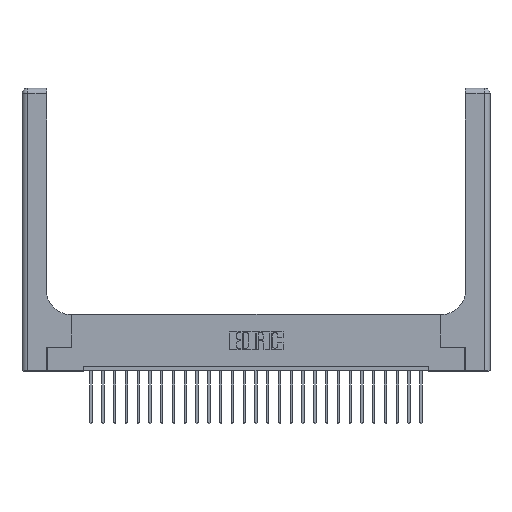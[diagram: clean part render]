
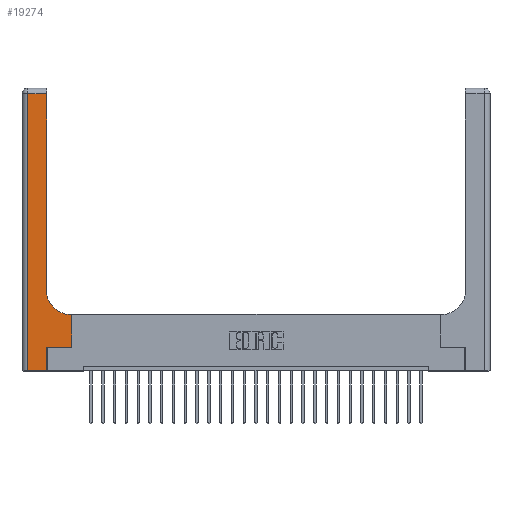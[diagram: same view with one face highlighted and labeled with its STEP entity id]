
A CAD part, top view. The second image highlights one B-rep face of the part: STEP entity #19274.
In plain terms, the highlighted planar face has unit normal (0, 0, 1).
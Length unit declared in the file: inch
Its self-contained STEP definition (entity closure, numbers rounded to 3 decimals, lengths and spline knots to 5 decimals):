
#1393 = CARTESIAN_POINT ( 'NONE',  ( 0., 0., 0.37 ) ) ;
#2733 = VERTEX_POINT ( 'NONE', #12878 ) ;
#2893 = EDGE_CURVE ( 'NONE', #7066, #9478, #19271, .T. ) ;
#3569 = CARTESIAN_POINT ( 'NONE',  ( 0., 2.94, 0.37 ) ) ;
#3649 = CARTESIAN_POINT ( 'NONE',  ( 0.51, 0.6, 0.37 ) ) ;
#3749 = EDGE_CURVE ( 'NONE', #22041, #7944, #23563, .T. ) ;
#4116 = CARTESIAN_POINT ( 'NONE',  ( 0., 3., 0.37 ) ) ;
#4631 = EDGE_CURVE ( 'NONE', #9478, #13828, #14816, .T. ) ;
#4731 = CARTESIAN_POINT ( 'NONE',  ( 0.528, 0.25, 0.37 ) ) ;
#5255 = LINE ( 'NONE', #1393, #12780 ) ;
#5630 = CIRCLE ( 'NONE', #20385, 0.25 ) ;
#5872 = DIRECTION ( 'NONE',  ( -1., 0., 0. ) ) ;
#5969 = DIRECTION ( 'NONE',  ( 0., 1., 0. ) ) ;
#6547 = EDGE_CURVE ( 'NONE', #13828, #21429, #15803, .T. ) ;
#6646 = DIRECTION ( 'NONE',  ( 1., 0., 0. ) ) ;
#6656 = CARTESIAN_POINT ( 'NONE',  ( 0.265, 0.25, 0.37 ) ) ;
#6867 = EDGE_CURVE ( 'NONE', #2733, #7066, #20140, .T. ) ;
#7066 = VERTEX_POINT ( 'NONE', #6656 ) ;
#7307 = DIRECTION ( 'NONE',  ( 1., 0., 0. ) ) ;
#7593 = CARTESIAN_POINT ( 'NONE',  ( 0.265, 0.25, 0.37 ) ) ;
#7886 = AXIS2_PLACEMENT_3D ( 'NONE', #4116, #15931, #19772 ) ;
#7944 = VERTEX_POINT ( 'NONE', #18975 ) ;
#8501 = ORIENTED_EDGE ( 'NONE', *, *, #2893, .T. ) ;
#8572 = CARTESIAN_POINT ( 'NONE',  ( 0.51, 0.85, 0.37 ) ) ;
#8751 = VECTOR ( 'NONE', #16295, 39.37008 ) ;
#9478 = VERTEX_POINT ( 'NONE', #4731 ) ;
#10160 = DIRECTION ( 'NONE',  ( -1., 0., 0. ) ) ;
#10286 = FACE_OUTER_BOUND ( 'NONE', #10480, .T. ) ;
#10480 = EDGE_LOOP ( 'NONE', ( #19720, #17516, #15039, #15432, #15821, #8501, #23586, #16377, #21951 ) ) ;
#10783 = VERTEX_POINT ( 'NONE', #24390 ) ;
#10808 = VECTOR ( 'NONE', #5969, 39.37008 ) ;
#11617 = VECTOR ( 'NONE', #14775, 39.37008 ) ;
#11956 = CARTESIAN_POINT ( 'NONE',  ( 0.26, 0.6, 0.37 ) ) ;
#12054 = CARTESIAN_POINT ( 'NONE',  ( 0.265, 0., 0.37 ) ) ;
#12780 = VECTOR ( 'NONE', #7307, 39.37008 ) ;
#12878 = CARTESIAN_POINT ( 'NONE',  ( 0.265, 0., 0.37 ) ) ;
#12920 = CARTESIAN_POINT ( 'NONE',  ( 0.528, 0.6, 0.37 ) ) ;
#13828 = VERTEX_POINT ( 'NONE', #12920 ) ;
#14417 = VECTOR ( 'NONE', #14699, 39.37008 ) ;
#14699 = DIRECTION ( 'NONE',  ( 0., 1., 0. ) ) ;
#14775 = DIRECTION ( 'NONE',  ( 0., -1., 0. ) ) ;
#14816 = LINE ( 'NONE', #16756, #14417 ) ;
#14889 = LINE ( 'NONE', #15014, #11617 ) ;
#15014 = CARTESIAN_POINT ( 'NONE',  ( 0.06, 3., 0.37 ) ) ;
#15039 = ORIENTED_EDGE ( 'NONE', *, *, #20365, .T. ) ;
#15304 = VECTOR ( 'NONE', #10160, 39.37008 ) ;
#15432 = ORIENTED_EDGE ( 'NONE', *, *, #24772, .T. ) ;
#15510 = LINE ( 'NONE', #3569, #15992 ) ;
#15803 = LINE ( 'NONE', #11956, #15304 ) ;
#15821 = ORIENTED_EDGE ( 'NONE', *, *, #6867, .T. ) ;
#15931 = DIRECTION ( 'NONE',  ( 0., 0., -1. ) ) ;
#15992 = VECTOR ( 'NONE', #5872, 39.37008 ) ;
#16295 = DIRECTION ( 'NONE',  ( 0., 1., 0. ) ) ;
#16377 = ORIENTED_EDGE ( 'NONE', *, *, #6547, .T. ) ;
#16421 = DIRECTION ( 'NONE',  ( 0., 0., -1. ) ) ;
#16756 = CARTESIAN_POINT ( 'NONE',  ( 0.528, 0.25, 0.37 ) ) ;
#17516 = ORIENTED_EDGE ( 'NONE', *, *, #17798, .T. ) ;
#17798 = EDGE_CURVE ( 'NONE', #7944, #17841, #15510, .T. ) ;
#17841 = VERTEX_POINT ( 'NONE', #23216 ) ;
#18975 = CARTESIAN_POINT ( 'NONE',  ( 0.26, 2.94, 0.37 ) ) ;
#19271 = LINE ( 'NONE', #7593, #23895 ) ;
#19274 = ADVANCED_FACE ( 'NONE', ( #10286 ), #21705, .F. ) ;
#19720 = ORIENTED_EDGE ( 'NONE', *, *, #3749, .T. ) ;
#19772 = DIRECTION ( 'NONE',  ( -1., 0., 0. ) ) ;
#20140 = LINE ( 'NONE', #12054, #8751 ) ;
#20302 = CARTESIAN_POINT ( 'NONE',  ( 0.26, 0.85, 0.37 ) ) ;
#20365 = EDGE_CURVE ( 'NONE', #17841, #10783, #14889, .T. ) ;
#20385 = AXIS2_PLACEMENT_3D ( 'NONE', #8572, #16421, #6646 ) ;
#21208 = DIRECTION ( 'NONE',  ( 1., 0., 0. ) ) ;
#21429 = VERTEX_POINT ( 'NONE', #3649 ) ;
#21705 = PLANE ( 'NONE',  #7886 ) ;
#21951 = ORIENTED_EDGE ( 'NONE', *, *, #25001, .T. ) ;
#22041 = VERTEX_POINT ( 'NONE', #20302 ) ;
#23216 = CARTESIAN_POINT ( 'NONE',  ( 0.06, 2.94, 0.37 ) ) ;
#23563 = LINE ( 'NONE', #23696, #10808 ) ;
#23586 = ORIENTED_EDGE ( 'NONE', *, *, #4631, .T. ) ;
#23696 = CARTESIAN_POINT ( 'NONE',  ( 0.26, 3., 0.37 ) ) ;
#23895 = VECTOR ( 'NONE', #21208, 39.37008 ) ;
#24390 = CARTESIAN_POINT ( 'NONE',  ( 0.06, 0., 0.37 ) ) ;
#24772 = EDGE_CURVE ( 'NONE', #10783, #2733, #5255, .T. ) ;
#25001 = EDGE_CURVE ( 'NONE', #21429, #22041, #5630, .T. ) ;
